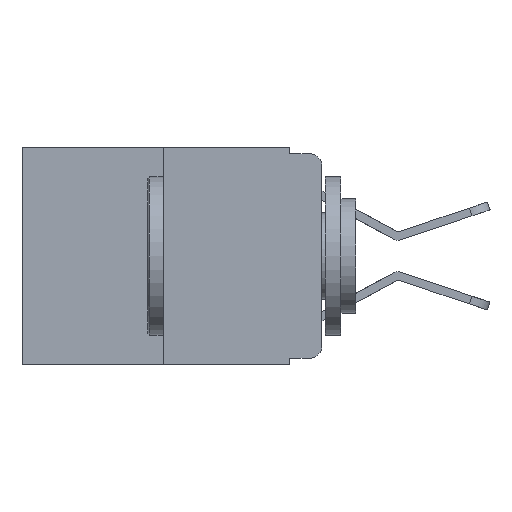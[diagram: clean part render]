
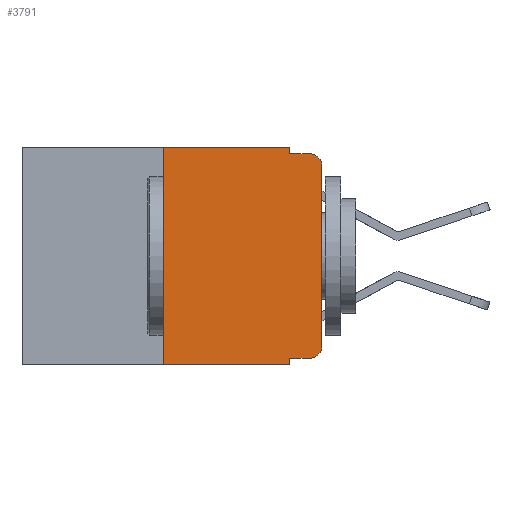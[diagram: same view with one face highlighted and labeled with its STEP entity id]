
A CAD part, left-side view. The second image highlights one B-rep face of the part: STEP entity #3791.
In plain terms, the highlighted planar face has unit normal (-1, 0, 0).
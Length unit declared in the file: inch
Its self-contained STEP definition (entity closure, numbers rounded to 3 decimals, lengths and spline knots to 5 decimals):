
#203 = VERTEX_POINT ( 'NONE', #15385 ) ;
#417 = VERTEX_POINT ( 'NONE', #15026 ) ;
#641 = DIRECTION ( 'NONE',  ( 0., 0., 1. ) ) ;
#741 = DIRECTION ( 'NONE',  ( 0., 0., -1. ) ) ;
#1114 = VERTEX_POINT ( 'NONE', #5350 ) ;
#1320 = DIRECTION ( 'NONE',  ( 0., -1., 0. ) ) ;
#1633 = CARTESIAN_POINT ( 'NONE',  ( 0., 0.051, -0.01 ) ) ;
#1765 = CARTESIAN_POINT ( 'NONE',  ( 0., 0.473, 0. ) ) ;
#1977 = DIRECTION ( 'NONE',  ( 0., 0., -1. ) ) ;
#2046 = CARTESIAN_POINT ( 'NONE',  ( 0., 0.051, -0.333 ) ) ;
#2441 = AXIS2_PLACEMENT_3D ( 'NONE', #6622, #9147, #9163 ) ;
#2527 = VERTEX_POINT ( 'NONE', #1633 ) ;
#2602 = ORIENTED_EDGE ( 'NONE', *, *, #10305, .F. ) ;
#2893 = VECTOR ( 'NONE', #641, 39.37008 ) ;
#3184 = ORIENTED_EDGE ( 'NONE', *, *, #7120, .T. ) ;
#3498 = VERTEX_POINT ( 'NONE', #13586 ) ;
#3576 = ORIENTED_EDGE ( 'NONE', *, *, #13413, .T. ) ;
#3657 = AXIS2_PLACEMENT_3D ( 'NONE', #5459, #13682, #6648 ) ;
#3790 = ORIENTED_EDGE ( 'NONE', *, *, #8745, .F. ) ;
#3791 = ADVANCED_FACE ( 'NONE', ( #8164 ), #13691, .F. ) ;
#3809 = VERTEX_POINT ( 'NONE', #7900 ) ;
#3833 = LINE ( 'NONE', #9638, #9820 ) ;
#4760 = CARTESIAN_POINT ( 'NONE',  ( 0., 0.051, -0.333 ) ) ;
#4835 = LINE ( 'NONE', #1765, #13835 ) ;
#4873 = CARTESIAN_POINT ( 'NONE',  ( 0., 0.02, -0.333 ) ) ;
#5350 = CARTESIAN_POINT ( 'NONE',  ( 0., 0., -0.313 ) ) ;
#5459 = CARTESIAN_POINT ( 'NONE',  ( 0., 0.02, -0.03 ) ) ;
#5468 = DIRECTION ( 'NONE',  ( 0., -1., 0. ) ) ;
#5821 = ORIENTED_EDGE ( 'NONE', *, *, #14629, .T. ) ;
#6210 = VERTEX_POINT ( 'NONE', #9583 ) ;
#6559 = CARTESIAN_POINT ( 'NONE',  ( 0., 0., 0. ) ) ;
#6622 = CARTESIAN_POINT ( 'NONE',  ( 0., 0.473, 0. ) ) ;
#6648 = DIRECTION ( 'NONE',  ( 0., 0., -1. ) ) ;
#7120 = EDGE_CURVE ( 'NONE', #9523, #1114, #8930, .T. ) ;
#7150 = ORIENTED_EDGE ( 'NONE', *, *, #12656, .T. ) ;
#7377 = LINE ( 'NONE', #8025, #12909 ) ;
#7411 = CARTESIAN_POINT ( 'NONE',  ( 0., 0.051, -0.01 ) ) ;
#7677 = AXIS2_PLACEMENT_3D ( 'NONE', #15052, #8113, #741 ) ;
#7887 = ORIENTED_EDGE ( 'NONE', *, *, #11126, .F. ) ;
#7900 = CARTESIAN_POINT ( 'NONE',  ( 0., 0., -0.03 ) ) ;
#7910 = EDGE_CURVE ( 'NONE', #11551, #9523, #14134, .T. ) ;
#8025 = CARTESIAN_POINT ( 'NONE',  ( 0., 0.051, 0. ) ) ;
#8113 = DIRECTION ( 'NONE',  ( -1., 0., 0. ) ) ;
#8164 = FACE_OUTER_BOUND ( 'NONE', #8229, .T. ) ;
#8229 = EDGE_LOOP ( 'NONE', ( #3576, #7150, #10310, #7887, #11405, #2602, #5821, #3790, #8844, #3184 ) ) ;
#8735 = VECTOR ( 'NONE', #13892, 39.37008 ) ;
#8745 = EDGE_CURVE ( 'NONE', #11551, #417, #7377, .T. ) ;
#8844 = ORIENTED_EDGE ( 'NONE', *, *, #7910, .T. ) ;
#8930 = CIRCLE ( 'NONE', #7677, 0.02 ) ;
#9073 = CARTESIAN_POINT ( 'NONE',  ( 0., 0.25, -0.343 ) ) ;
#9147 = DIRECTION ( 'NONE',  ( 1., 0., 0. ) ) ;
#9163 = DIRECTION ( 'NONE',  ( 0., 0., -1. ) ) ;
#9523 = VERTEX_POINT ( 'NONE', #4873 ) ;
#9583 = CARTESIAN_POINT ( 'NONE',  ( 0., 0.051, 0. ) ) ;
#9638 = CARTESIAN_POINT ( 'NONE',  ( 0., 0.473, -0.343 ) ) ;
#9761 = VECTOR ( 'NONE', #13606, 39.37008 ) ;
#9820 = VECTOR ( 'NONE', #10834, 39.37008 ) ;
#10228 = EDGE_CURVE ( 'NONE', #3498, #6210, #4835, .T. ) ;
#10305 = EDGE_CURVE ( 'NONE', #14123, #3498, #15418, .T. ) ;
#10310 = ORIENTED_EDGE ( 'NONE', *, *, #11886, .F. ) ;
#10772 = VECTOR ( 'NONE', #14131, 39.37008 ) ;
#10834 = DIRECTION ( 'NONE',  ( 0., -1., 0. ) ) ;
#11126 = EDGE_CURVE ( 'NONE', #6210, #2527, #14860, .T. ) ;
#11284 = LINE ( 'NONE', #7411, #11630 ) ;
#11405 = ORIENTED_EDGE ( 'NONE', *, *, #10228, .F. ) ;
#11551 = VERTEX_POINT ( 'NONE', #2046 ) ;
#11630 = VECTOR ( 'NONE', #1320, 39.37008 ) ;
#11886 = EDGE_CURVE ( 'NONE', #2527, #203, #11284, .T. ) ;
#12656 = EDGE_CURVE ( 'NONE', #3809, #203, #13406, .T. ) ;
#12797 = CARTESIAN_POINT ( 'NONE',  ( 0., 0.051, 0. ) ) ;
#12909 = VECTOR ( 'NONE', #1977, 39.37008 ) ;
#13213 = LINE ( 'NONE', #6559, #9761 ) ;
#13406 = CIRCLE ( 'NONE', #3657, 0.02 ) ;
#13413 = EDGE_CURVE ( 'NONE', #1114, #3809, #13213, .T. ) ;
#13586 = CARTESIAN_POINT ( 'NONE',  ( 0., 0.25, 0. ) ) ;
#13606 = DIRECTION ( 'NONE',  ( 0., 0., 1. ) ) ;
#13682 = DIRECTION ( 'NONE',  ( -1., 0., 0. ) ) ;
#13691 = PLANE ( 'NONE',  #2441 ) ;
#13835 = VECTOR ( 'NONE', #5468, 39.37008 ) ;
#13892 = DIRECTION ( 'NONE',  ( 0., 0., -1. ) ) ;
#14123 = VERTEX_POINT ( 'NONE', #9073 ) ;
#14131 = DIRECTION ( 'NONE',  ( 0., -1., 0. ) ) ;
#14134 = LINE ( 'NONE', #4760, #10772 ) ;
#14629 = EDGE_CURVE ( 'NONE', #14123, #417, #3833, .T. ) ;
#14860 = LINE ( 'NONE', #12797, #8735 ) ;
#14941 = CARTESIAN_POINT ( 'NONE',  ( 0., 0.25, 0. ) ) ;
#15026 = CARTESIAN_POINT ( 'NONE',  ( 0., 0.051, -0.343 ) ) ;
#15052 = CARTESIAN_POINT ( 'NONE',  ( 0., 0.02, -0.313 ) ) ;
#15385 = CARTESIAN_POINT ( 'NONE',  ( 0., 0.02, -0.01 ) ) ;
#15418 = LINE ( 'NONE', #14941, #2893 ) ;
